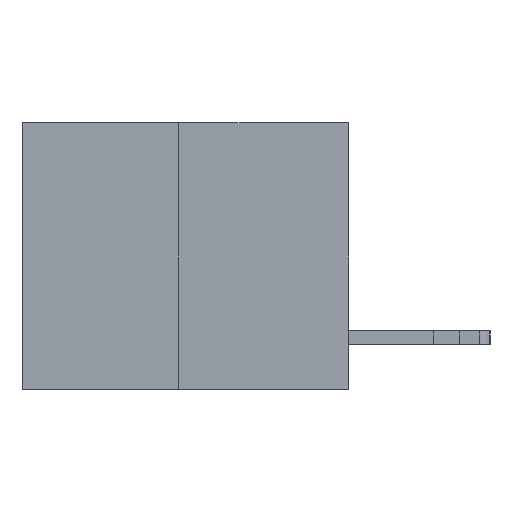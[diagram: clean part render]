
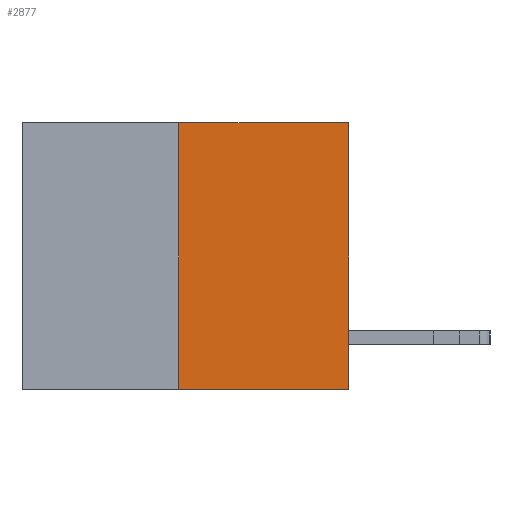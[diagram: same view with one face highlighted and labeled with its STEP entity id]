
A CAD part, left-side view. The second image highlights one B-rep face of the part: STEP entity #2877.
In plain terms, the highlighted planar face has unit normal (-1, 0, 0).
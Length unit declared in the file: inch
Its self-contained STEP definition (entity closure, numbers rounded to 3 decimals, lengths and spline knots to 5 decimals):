
#1155 = DIRECTION ( 'NONE',  ( 0., 0., 1. ) ) ;
#1472 = VECTOR ( 'NONE', #20959, 39.37008 ) ;
#2660 = EDGE_CURVE ( 'NONE', #18077, #12281, #22331, .T. ) ;
#2877 = ADVANCED_FACE ( 'NONE', ( #16820 ), #18186, .F. ) ;
#4467 = CARTESIAN_POINT ( 'NONE',  ( 0., 0., -0.49 ) ) ;
#4868 = DIRECTION ( 'NONE',  ( 0., 0., -1. ) ) ;
#5582 = EDGE_LOOP ( 'NONE', ( #27293, #13695, #11461, #24983 ) ) ;
#7079 = EDGE_CURVE ( 'NONE', #11367, #12281, #12023, .T. ) ;
#7291 = CARTESIAN_POINT ( 'NONE',  ( 0., 0.6, 0. ) ) ;
#7601 = DIRECTION ( 'NONE',  ( 0., 0., 1. ) ) ;
#9340 = CARTESIAN_POINT ( 'NONE',  ( 0., 0.312, -0.49 ) ) ;
#11367 = VERTEX_POINT ( 'NONE', #4467 ) ;
#11461 = ORIENTED_EDGE ( 'NONE', *, *, #7079, .T. ) ;
#12023 = LINE ( 'NONE', #14115, #14854 ) ;
#12281 = VERTEX_POINT ( 'NONE', #15536 ) ;
#12469 = DIRECTION ( 'NONE',  ( 0., -1., 0. ) ) ;
#12515 = CARTESIAN_POINT ( 'NONE',  ( 0., 0.312, 0. ) ) ;
#13036 = LINE ( 'NONE', #23755, #23084 ) ;
#13695 = ORIENTED_EDGE ( 'NONE', *, *, #28161, .T. ) ;
#13821 = DIRECTION ( 'NONE',  ( 1., 0., 0. ) ) ;
#14115 = CARTESIAN_POINT ( 'NONE',  ( 0., 0., 0. ) ) ;
#14167 = CARTESIAN_POINT ( 'NONE',  ( 0., 0.6, 0. ) ) ;
#14527 = CARTESIAN_POINT ( 'NONE',  ( 0., 0.312, -0.49 ) ) ;
#14854 = VECTOR ( 'NONE', #7601, 39.37008 ) ;
#15536 = CARTESIAN_POINT ( 'NONE',  ( 0., 0., 0. ) ) ;
#16820 = FACE_OUTER_BOUND ( 'NONE', #5582, .T. ) ;
#18077 = VERTEX_POINT ( 'NONE', #12515 ) ;
#18186 = PLANE ( 'NONE',  #21778 ) ;
#18374 = LINE ( 'NONE', #14527, #20812 ) ;
#20812 = VECTOR ( 'NONE', #1155, 39.37008 ) ;
#20959 = DIRECTION ( 'NONE',  ( 0., -1., 0. ) ) ;
#21778 = AXIS2_PLACEMENT_3D ( 'NONE', #7291, #13821, #4868 ) ;
#22331 = LINE ( 'NONE', #14167, #1472 ) ;
#23084 = VECTOR ( 'NONE', #12469, 39.37008 ) ;
#23755 = CARTESIAN_POINT ( 'NONE',  ( 0., 0.6, -0.49 ) ) ;
#24983 = ORIENTED_EDGE ( 'NONE', *, *, #2660, .F. ) ;
#26302 = EDGE_CURVE ( 'NONE', #27840, #18077, #18374, .T. ) ;
#27293 = ORIENTED_EDGE ( 'NONE', *, *, #26302, .F. ) ;
#27840 = VERTEX_POINT ( 'NONE', #9340 ) ;
#28161 = EDGE_CURVE ( 'NONE', #27840, #11367, #13036, .T. ) ;
